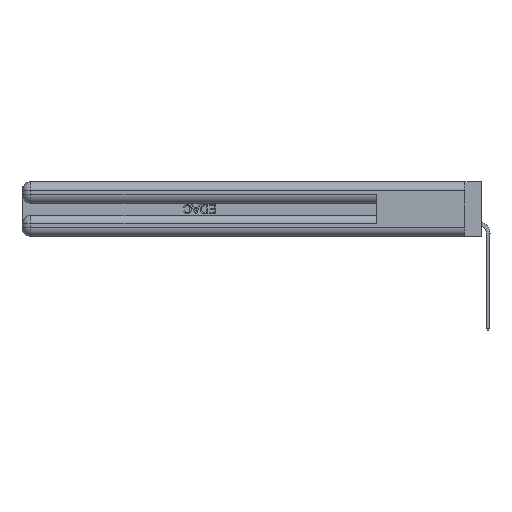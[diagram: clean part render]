
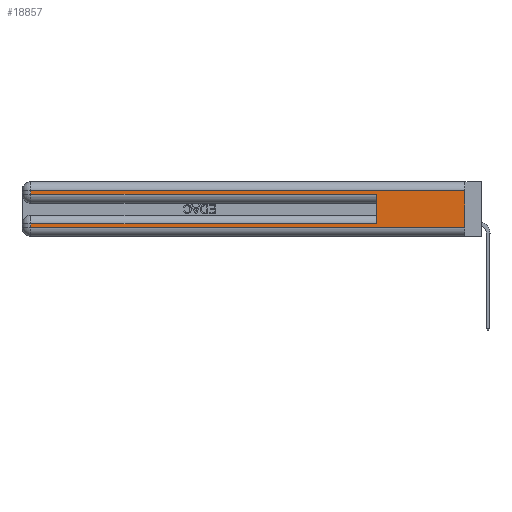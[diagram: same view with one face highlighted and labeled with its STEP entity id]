
A CAD part, left-side view. The second image highlights one B-rep face of the part: STEP entity #18857.
In plain terms, the highlighted planar face has unit normal (-1, 0, 0).
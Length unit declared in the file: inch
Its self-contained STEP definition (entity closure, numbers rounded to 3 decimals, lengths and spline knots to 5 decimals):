
#19 = ORIENTED_EDGE ( 'NONE', *, *, #48412, .T. ) ;
#158 = VERTEX_POINT ( 'NONE', #48707 ) ;
#536 = VERTEX_POINT ( 'NONE', #43438 ) ;
#4885 = CARTESIAN_POINT ( 'NONE',  ( 0., 0.6, 0.145 ) ) ;
#4992 = EDGE_CURVE ( 'NONE', #158, #536, #45337, .T. ) ;
#5597 = DIRECTION ( 'NONE',  ( 1., 0., 0. ) ) ;
#5862 = CARTESIAN_POINT ( 'NONE',  ( 0., 2.94, 0.085 ) ) ;
#5886 = CARTESIAN_POINT ( 'NONE',  ( 0., 0., 0.37 ) ) ;
#6063 = LINE ( 'NONE', #31049, #21100 ) ;
#7001 = EDGE_CURVE ( 'NONE', #22221, #536, #6063, .T. ) ;
#9740 = LINE ( 'NONE', #49211, #48468 ) ;
#10394 = CARTESIAN_POINT ( 'NONE',  ( 0., 0., 0.31 ) ) ;
#10411 = CARTESIAN_POINT ( 'NONE',  ( 0., 0., 0.085 ) ) ;
#11143 = EDGE_CURVE ( 'NONE', #51216, #43021, #40631, .T. ) ;
#13054 = DIRECTION ( 'NONE',  ( 0., -1., 0. ) ) ;
#14912 = DIRECTION ( 'NONE',  ( 0., -1., 0. ) ) ;
#15973 = CARTESIAN_POINT ( 'NONE',  ( 0., 0., 0.31 ) ) ;
#15982 = CARTESIAN_POINT ( 'NONE',  ( 0., 2.94, 0.37 ) ) ;
#16680 = VECTOR ( 'NONE', #32896, 39.37008 ) ;
#17019 = ORIENTED_EDGE ( 'NONE', *, *, #51672, .F. ) ;
#17577 = PLANE ( 'NONE',  #40559 ) ;
#18375 = DIRECTION ( 'NONE',  ( 0., 0., -1. ) ) ;
#18857 = ADVANCED_FACE ( 'NONE', ( #45321 ), #17577, .F. ) ;
#19036 = ORIENTED_EDGE ( 'NONE', *, *, #27159, .T. ) ;
#21100 = VECTOR ( 'NONE', #14912, 39.37008 ) ;
#21260 = VECTOR ( 'NONE', #45603, 39.37008 ) ;
#21590 = EDGE_CURVE ( 'NONE', #158, #32238, #41889, .T. ) ;
#22197 = ORIENTED_EDGE ( 'NONE', *, *, #21590, .T. ) ;
#22221 = VERTEX_POINT ( 'NONE', #48442 ) ;
#25157 = VERTEX_POINT ( 'NONE', #31356 ) ;
#27159 = EDGE_CURVE ( 'NONE', #25157, #34946, #9740, .T. ) ;
#28190 = DIRECTION ( 'NONE',  ( 0., 0., -1. ) ) ;
#29245 = CARTESIAN_POINT ( 'NONE',  ( 0., 0., 0.37 ) ) ;
#29331 = VECTOR ( 'NONE', #39653, 39.37008 ) ;
#29846 = VECTOR ( 'NONE', #28190, 39.37008 ) ;
#30005 = ORIENTED_EDGE ( 'NONE', *, *, #4992, .F. ) ;
#30237 = ORIENTED_EDGE ( 'NONE', *, *, #7001, .T. ) ;
#31049 = CARTESIAN_POINT ( 'NONE',  ( 0., 0., 0.285 ) ) ;
#31356 = CARTESIAN_POINT ( 'NONE',  ( 0., 2.94, 0.06 ) ) ;
#31428 = LINE ( 'NONE', #5886, #47601 ) ;
#31954 = CARTESIAN_POINT ( 'NONE',  ( 0., 0., 0.06 ) ) ;
#32238 = VERTEX_POINT ( 'NONE', #5862 ) ;
#32573 = CARTESIAN_POINT ( 'NONE',  ( 0., 2.94, 0.31 ) ) ;
#32896 = DIRECTION ( 'NONE',  ( 0., 0., 1. ) ) ;
#33470 = ORIENTED_EDGE ( 'NONE', *, *, #11143, .T. ) ;
#34916 = DIRECTION ( 'NONE',  ( 0., 1., 0. ) ) ;
#34945 = EDGE_CURVE ( 'NONE', #32238, #25157, #36781, .T. ) ;
#34946 = VERTEX_POINT ( 'NONE', #31954 ) ;
#36781 = LINE ( 'NONE', #39983, #29331 ) ;
#36872 = VECTOR ( 'NONE', #34916, 39.37008 ) ;
#39653 = DIRECTION ( 'NONE',  ( 0., 0., -1. ) ) ;
#39983 = CARTESIAN_POINT ( 'NONE',  ( 0., 2.94, 0.37 ) ) ;
#40559 = AXIS2_PLACEMENT_3D ( 'NONE', #29245, #5597, #49525 ) ;
#40631 = LINE ( 'NONE', #10394, #21260 ) ;
#41889 = LINE ( 'NONE', #10411, #36872 ) ;
#42310 = LINE ( 'NONE', #15982, #29846 ) ;
#43021 = VERTEX_POINT ( 'NONE', #32573 ) ;
#43438 = CARTESIAN_POINT ( 'NONE',  ( 0., 0.6, 0.285 ) ) ;
#45321 = FACE_OUTER_BOUND ( 'NONE', #51816, .T. ) ;
#45337 = LINE ( 'NONE', #4885, #16680 ) ;
#45603 = DIRECTION ( 'NONE',  ( 0., 1., 0. ) ) ;
#47601 = VECTOR ( 'NONE', #18375, 39.37008 ) ;
#48412 = EDGE_CURVE ( 'NONE', #43021, #22221, #42310, .T. ) ;
#48442 = CARTESIAN_POINT ( 'NONE',  ( 0., 2.94, 0.285 ) ) ;
#48468 = VECTOR ( 'NONE', #13054, 39.37008 ) ;
#48586 = ORIENTED_EDGE ( 'NONE', *, *, #34945, .T. ) ;
#48707 = CARTESIAN_POINT ( 'NONE',  ( 0., 0.6, 0.085 ) ) ;
#49211 = CARTESIAN_POINT ( 'NONE',  ( 0., 0., 0.06 ) ) ;
#49525 = DIRECTION ( 'NONE',  ( 0., 0., -1. ) ) ;
#51216 = VERTEX_POINT ( 'NONE', #15973 ) ;
#51672 = EDGE_CURVE ( 'NONE', #51216, #34946, #31428, .T. ) ;
#51816 = EDGE_LOOP ( 'NONE', ( #17019, #33470, #19, #30237, #30005, #22197, #48586, #19036 ) ) ;
